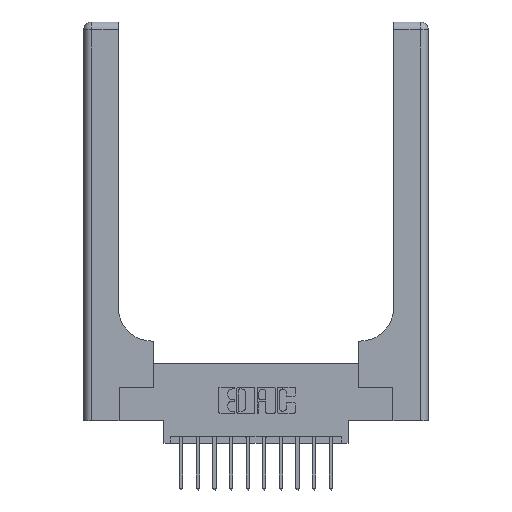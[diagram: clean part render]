
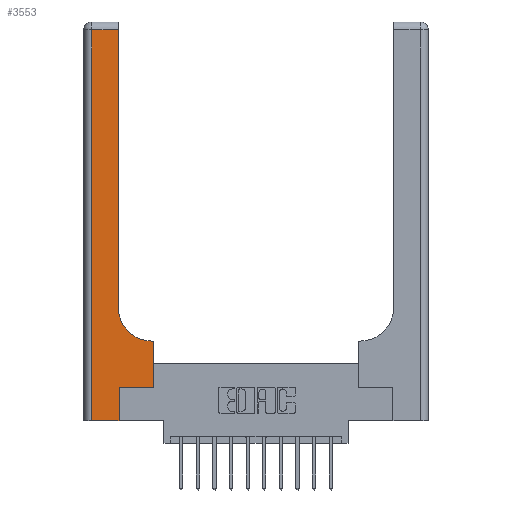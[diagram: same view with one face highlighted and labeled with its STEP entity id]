
A CAD part, top view. The second image highlights one B-rep face of the part: STEP entity #3553.
In plain terms, the highlighted planar face has unit normal (0, 0, 1).
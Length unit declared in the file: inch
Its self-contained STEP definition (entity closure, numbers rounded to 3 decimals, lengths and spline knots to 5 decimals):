
#364 = DIRECTION ( 'NONE',  ( 1., 0., 0. ) ) ;
#834 = VERTEX_POINT ( 'NONE', #3215 ) ;
#842 = EDGE_CURVE ( 'NONE', #5763, #12737, #9247, .T. ) ;
#1046 = CARTESIAN_POINT ( 'NONE',  ( 0.26, 0.6, 0.37 ) ) ;
#1060 = VECTOR ( 'NONE', #6927, 39.37008 ) ;
#1351 = VECTOR ( 'NONE', #4474, 39.37008 ) ;
#1436 = EDGE_CURVE ( 'NONE', #2785, #834, #1737, .T. ) ;
#1737 = LINE ( 'NONE', #11972, #1351 ) ;
#1976 = EDGE_CURVE ( 'NONE', #15434, #7314, #7652, .T. ) ;
#2208 = LINE ( 'NONE', #1046, #14747 ) ;
#2241 = EDGE_CURVE ( 'NONE', #5586, #15434, #7443, .T. ) ;
#2711 = LINE ( 'NONE', #10682, #9021 ) ;
#2785 = VERTEX_POINT ( 'NONE', #6584 ) ;
#3112 = ORIENTED_EDGE ( 'NONE', *, *, #8012, .T. ) ;
#3166 = DIRECTION ( 'NONE',  ( 0., -1., 0. ) ) ;
#3177 = VECTOR ( 'NONE', #15993, 39.37008 ) ;
#3215 = CARTESIAN_POINT ( 'NONE',  ( 0.265, 0.25, 0.37 ) ) ;
#3239 = DIRECTION ( 'NONE',  ( 0., 1., 0. ) ) ;
#3553 = ADVANCED_FACE ( 'NONE', ( #9194 ), #14387, .F. ) ;
#3875 = VECTOR ( 'NONE', #8121, 39.37008 ) ;
#4474 = DIRECTION ( 'NONE',  ( 0., 1., 0. ) ) ;
#4696 = VECTOR ( 'NONE', #3239, 39.37008 ) ;
#5170 = CARTESIAN_POINT ( 'NONE',  ( 0.528, 0.25, 0.37 ) ) ;
#5586 = VERTEX_POINT ( 'NONE', #6125 ) ;
#5763 = VERTEX_POINT ( 'NONE', #5170 ) ;
#5914 = VECTOR ( 'NONE', #8304, 39.37008 ) ;
#6125 = CARTESIAN_POINT ( 'NONE',  ( 0.51, 0.6, 0.37 ) ) ;
#6266 = ORIENTED_EDGE ( 'NONE', *, *, #10113, .T. ) ;
#6584 = CARTESIAN_POINT ( 'NONE',  ( 0.265, 0., 0.37 ) ) ;
#6697 = AXIS2_PLACEMENT_3D ( 'NONE', #15369, #7918, #364 ) ;
#6927 = DIRECTION ( 'NONE',  ( 1., 0., 0. ) ) ;
#6939 = DIRECTION ( 'NONE',  ( 0., 0., -1. ) ) ;
#7004 = CARTESIAN_POINT ( 'NONE',  ( 0.26, 3., 0.37 ) ) ;
#7041 = CARTESIAN_POINT ( 'NONE',  ( 0.528, 0.25, 0.37 ) ) ;
#7314 = VERTEX_POINT ( 'NONE', #10912 ) ;
#7443 = CIRCLE ( 'NONE', #6697, 0.25 ) ;
#7652 = LINE ( 'NONE', #7004, #4696 ) ;
#7738 = CARTESIAN_POINT ( 'NONE',  ( 0.528, 0.6, 0.37 ) ) ;
#7786 = LINE ( 'NONE', #13156, #1060 ) ;
#7918 = DIRECTION ( 'NONE',  ( 0., 0., -1. ) ) ;
#8012 = EDGE_CURVE ( 'NONE', #13963, #2785, #8023, .T. ) ;
#8023 = LINE ( 'NONE', #14313, #3875 ) ;
#8121 = DIRECTION ( 'NONE',  ( 1., 0., 0. ) ) ;
#8145 = CARTESIAN_POINT ( 'NONE',  ( 0., 3., 0.37 ) ) ;
#8304 = DIRECTION ( 'NONE',  ( 0., 1., 0. ) ) ;
#8546 = CARTESIAN_POINT ( 'NONE',  ( 0., 2.94, 0.37 ) ) ;
#8803 = AXIS2_PLACEMENT_3D ( 'NONE', #8145, #6939, #15653 ) ;
#9021 = VECTOR ( 'NONE', #3166, 39.37008 ) ;
#9127 = CARTESIAN_POINT ( 'NONE',  ( 0.06, 2.94, 0.37 ) ) ;
#9194 = FACE_OUTER_BOUND ( 'NONE', #12061, .T. ) ;
#9204 = EDGE_CURVE ( 'NONE', #834, #5763, #7786, .T. ) ;
#9247 = LINE ( 'NONE', #7041, #5914 ) ;
#9872 = LINE ( 'NONE', #8546, #3177 ) ;
#9898 = DIRECTION ( 'NONE',  ( -1., 0., 0. ) ) ;
#9965 = ORIENTED_EDGE ( 'NONE', *, *, #9204, .T. ) ;
#10044 = CARTESIAN_POINT ( 'NONE',  ( 0.06, 0., 0.37 ) ) ;
#10113 = EDGE_CURVE ( 'NONE', #12737, #5586, #2208, .T. ) ;
#10529 = ORIENTED_EDGE ( 'NONE', *, *, #15554, .T. ) ;
#10682 = CARTESIAN_POINT ( 'NONE',  ( 0.06, 3., 0.37 ) ) ;
#10730 = EDGE_CURVE ( 'NONE', #7314, #15342, #9872, .T. ) ;
#10912 = CARTESIAN_POINT ( 'NONE',  ( 0.26, 2.94, 0.37 ) ) ;
#11424 = ORIENTED_EDGE ( 'NONE', *, *, #842, .T. ) ;
#11510 = ORIENTED_EDGE ( 'NONE', *, *, #1436, .T. ) ;
#11972 = CARTESIAN_POINT ( 'NONE',  ( 0.265, 0., 0.37 ) ) ;
#12061 = EDGE_LOOP ( 'NONE', ( #14833, #12232, #10529, #3112, #11510, #9965, #11424, #6266, #14285 ) ) ;
#12232 = ORIENTED_EDGE ( 'NONE', *, *, #10730, .T. ) ;
#12737 = VERTEX_POINT ( 'NONE', #7738 ) ;
#13156 = CARTESIAN_POINT ( 'NONE',  ( 0.265, 0.25, 0.37 ) ) ;
#13963 = VERTEX_POINT ( 'NONE', #10044 ) ;
#14124 = CARTESIAN_POINT ( 'NONE',  ( 0.26, 0.85, 0.37 ) ) ;
#14285 = ORIENTED_EDGE ( 'NONE', *, *, #2241, .T. ) ;
#14313 = CARTESIAN_POINT ( 'NONE',  ( 0., 0., 0.37 ) ) ;
#14387 = PLANE ( 'NONE',  #8803 ) ;
#14747 = VECTOR ( 'NONE', #9898, 39.37008 ) ;
#14833 = ORIENTED_EDGE ( 'NONE', *, *, #1976, .T. ) ;
#15342 = VERTEX_POINT ( 'NONE', #9127 ) ;
#15369 = CARTESIAN_POINT ( 'NONE',  ( 0.51, 0.85, 0.37 ) ) ;
#15434 = VERTEX_POINT ( 'NONE', #14124 ) ;
#15554 = EDGE_CURVE ( 'NONE', #15342, #13963, #2711, .T. ) ;
#15653 = DIRECTION ( 'NONE',  ( -1., 0., 0. ) ) ;
#15993 = DIRECTION ( 'NONE',  ( -1., 0., 0. ) ) ;
